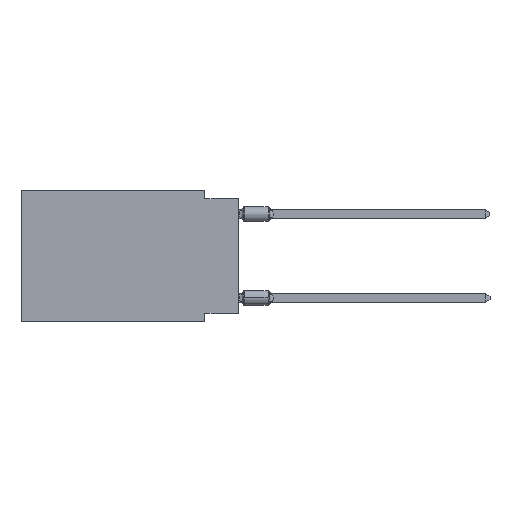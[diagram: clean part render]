
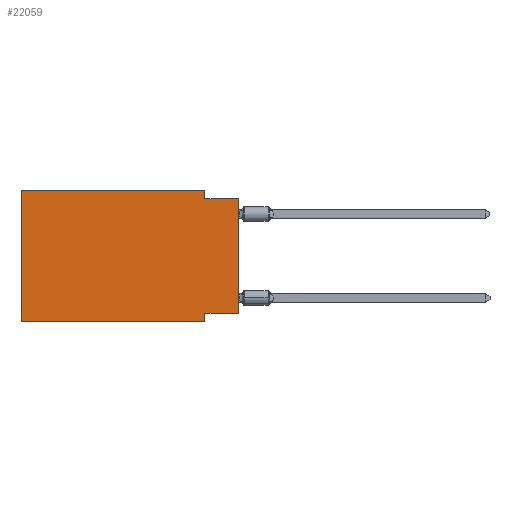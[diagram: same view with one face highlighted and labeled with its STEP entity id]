
A CAD part, left-side view. The second image highlights one B-rep face of the part: STEP entity #22059.
In plain terms, the highlighted planar face has unit normal (-1, 0, 0).
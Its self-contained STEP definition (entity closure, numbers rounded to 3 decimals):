
#11 = CARTESIAN_POINT ( 'NONE',  ( 0., 2.54, -9.906 ) ) ;
#489 = DIRECTION ( 'NONE',  ( 0., 0., 1. ) ) ;
#852 = ORIENTED_EDGE ( 'NONE', *, *, #7966, .T. ) ;
#1581 = DIRECTION ( 'NONE',  ( 0., 0., -1. ) ) ;
#3120 = CARTESIAN_POINT ( 'NONE',  ( 0., 2.54, -9.271 ) ) ;
#5008 = ORIENTED_EDGE ( 'NONE', *, *, #26381, .F. ) ;
#5261 = ORIENTED_EDGE ( 'NONE', *, *, #18051, .T. ) ;
#5540 = VERTEX_POINT ( 'NONE', #9622 ) ;
#6523 = CARTESIAN_POINT ( 'NONE',  ( 0., 2.54, -0.635 ) ) ;
#6654 = LINE ( 'NONE', #18420, #10212 ) ;
#7947 = ORIENTED_EDGE ( 'NONE', *, *, #29141, .F. ) ;
#7966 = EDGE_CURVE ( 'NONE', #36670, #5540, #14501, .T. ) ;
#8130 = PLANE ( 'NONE',  #35451 ) ;
#9477 = VECTOR ( 'NONE', #21781, 1000. ) ;
#9622 = CARTESIAN_POINT ( 'NONE',  ( 0., 2.54, -9.906 ) ) ;
#10212 = VECTOR ( 'NONE', #489, 1000. ) ;
#12605 = VECTOR ( 'NONE', #23194, 1000. ) ;
#13540 = LINE ( 'NONE', #28627, #35992 ) ;
#13598 = VERTEX_POINT ( 'NONE', #17527 ) ;
#13803 = LINE ( 'NONE', #37413, #34169 ) ;
#14501 = LINE ( 'NONE', #35769, #33557 ) ;
#14659 = LINE ( 'NONE', #11, #12605 ) ;
#15844 = LINE ( 'NONE', #27646, #23921 ) ;
#16431 = CARTESIAN_POINT ( 'NONE',  ( 0., 16.383, 0. ) ) ;
#17527 = CARTESIAN_POINT ( 'NONE',  ( 0., 0., -9.271 ) ) ;
#17605 = VERTEX_POINT ( 'NONE', #6523 ) ;
#18051 = EDGE_CURVE ( 'NONE', #13598, #33516, #13540, .T. ) ;
#18420 = CARTESIAN_POINT ( 'NONE',  ( 0., 16.383, 0. ) ) ;
#20539 = EDGE_CURVE ( 'NONE', #27370, #22857, #13803, .T. ) ;
#20545 = CARTESIAN_POINT ( 'NONE',  ( 0., 2.54, 0. ) ) ;
#20807 = CARTESIAN_POINT ( 'NONE',  ( 0., 0., -0.635 ) ) ;
#21058 = EDGE_CURVE ( 'NONE', #25131, #5540, #14659, .T. ) ;
#21781 = DIRECTION ( 'NONE',  ( 0., 1., 0. ) ) ;
#22059 = ADVANCED_FACE ( 'NONE', ( #25521 ), #8130, .F. ) ;
#22561 = LINE ( 'NONE', #24882, #9477 ) ;
#22857 = VERTEX_POINT ( 'NONE', #20545 ) ;
#23006 = ORIENTED_EDGE ( 'NONE', *, *, #31405, .F. ) ;
#23194 = DIRECTION ( 'NONE',  ( 0., 0., -1. ) ) ;
#23218 = EDGE_CURVE ( 'NONE', #17605, #33516, #26135, .T. ) ;
#23921 = VECTOR ( 'NONE', #1581, 1000. ) ;
#24882 = CARTESIAN_POINT ( 'NONE',  ( 0., 0., -9.271 ) ) ;
#25131 = VERTEX_POINT ( 'NONE', #3120 ) ;
#25345 = DIRECTION ( 'NONE',  ( 0., 0., 1. ) ) ;
#25521 = FACE_OUTER_BOUND ( 'NONE', #30358, .T. ) ;
#25609 = DIRECTION ( 'NONE',  ( 0., -1., 0. ) ) ;
#25928 = CARTESIAN_POINT ( 'NONE',  ( 0., 16.383, -9.906 ) ) ;
#26135 = LINE ( 'NONE', #32688, #29417 ) ;
#26381 = EDGE_CURVE ( 'NONE', #13598, #25131, #22561, .T. ) ;
#27370 = VERTEX_POINT ( 'NONE', #29212 ) ;
#27646 = CARTESIAN_POINT ( 'NONE',  ( 0., 2.54, 0. ) ) ;
#28239 = DIRECTION ( 'NONE',  ( 0., 0., -1. ) ) ;
#28627 = CARTESIAN_POINT ( 'NONE',  ( 0., 0., 0. ) ) ;
#29141 = EDGE_CURVE ( 'NONE', #36670, #27370, #6654, .T. ) ;
#29212 = CARTESIAN_POINT ( 'NONE',  ( 0., 16.383, 0. ) ) ;
#29417 = VECTOR ( 'NONE', #38121, 1000. ) ;
#30358 = EDGE_LOOP ( 'NONE', ( #5261, #36447, #23006, #36684, #7947, #852, #36598, #5008 ) ) ;
#31405 = EDGE_CURVE ( 'NONE', #22857, #17605, #15844, .T. ) ;
#32688 = CARTESIAN_POINT ( 'NONE',  ( 0., 0., -0.635 ) ) ;
#33516 = VERTEX_POINT ( 'NONE', #20807 ) ;
#33557 = VECTOR ( 'NONE', #38103, 1000. ) ;
#34169 = VECTOR ( 'NONE', #25609, 1000. ) ;
#35451 = AXIS2_PLACEMENT_3D ( 'NONE', #16431, #37126, #28239 ) ;
#35769 = CARTESIAN_POINT ( 'NONE',  ( 0., 16.383, -9.906 ) ) ;
#35992 = VECTOR ( 'NONE', #25345, 1000. ) ;
#36447 = ORIENTED_EDGE ( 'NONE', *, *, #23218, .F. ) ;
#36598 = ORIENTED_EDGE ( 'NONE', *, *, #21058, .F. ) ;
#36670 = VERTEX_POINT ( 'NONE', #25928 ) ;
#36684 = ORIENTED_EDGE ( 'NONE', *, *, #20539, .F. ) ;
#37126 = DIRECTION ( 'NONE',  ( 1., 0., 0. ) ) ;
#37413 = CARTESIAN_POINT ( 'NONE',  ( 0., 16.383, 0. ) ) ;
#38103 = DIRECTION ( 'NONE',  ( 0., -1., 0. ) ) ;
#38121 = DIRECTION ( 'NONE',  ( 0., -1., 0. ) ) ;
